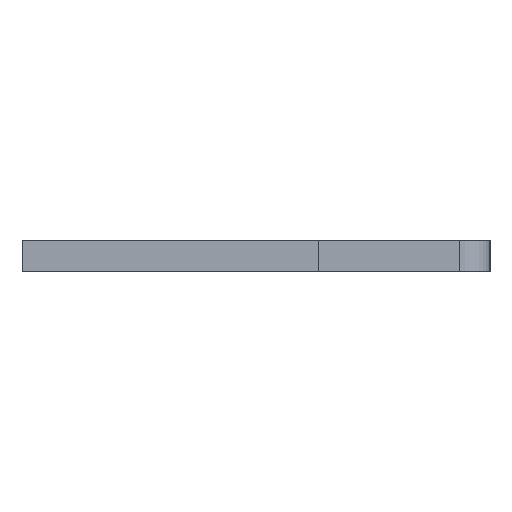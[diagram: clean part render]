
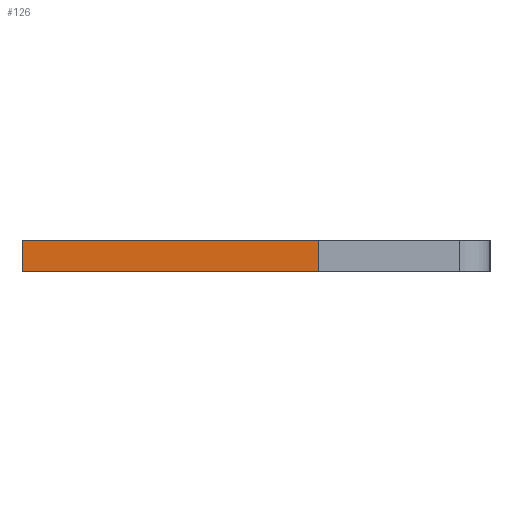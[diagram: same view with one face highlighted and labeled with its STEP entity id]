
A CAD part, left-side view. The second image highlights one B-rep face of the part: STEP entity #126.
In plain terms, the highlighted face is planar.
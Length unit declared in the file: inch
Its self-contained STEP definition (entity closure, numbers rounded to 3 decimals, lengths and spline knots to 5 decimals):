
#49 = VERTEX_POINT ( 'NONE', #751 ) ;
#65 = VECTOR ( 'NONE', #661, 39.37008 ) ;
#108 = ORIENTED_EDGE ( 'NONE', *, *, #788, .T. ) ;
#120 = PLANE ( 'NONE',  #532 ) ;
#126 = ADVANCED_FACE ( 'NONE', ( #1208 ), #120, .F. ) ;
#203 = EDGE_CURVE ( 'NONE', #691, #882, #754, .T. ) ;
#280 = CARTESIAN_POINT ( 'NONE',  ( 0.01, 0.15, -0.04 ) ) ;
#299 = CARTESIAN_POINT ( 'NONE',  ( -0.01, -0.04, -0.04 ) ) ;
#366 = ORIENTED_EDGE ( 'NONE', *, *, #372, .F. ) ;
#372 = EDGE_CURVE ( 'NONE', #1497, #882, #435, .T. ) ;
#435 = LINE ( 'NONE', #922, #771 ) ;
#532 = AXIS2_PLACEMENT_3D ( 'NONE', #910, #1214, #1453 ) ;
#661 = DIRECTION ( 'NONE',  ( 0., 1., 0. ) ) ;
#691 = VERTEX_POINT ( 'NONE', #299 ) ;
#693 = DIRECTION ( 'NONE',  ( -1., 0., 0. ) ) ;
#713 = EDGE_LOOP ( 'NONE', ( #1251, #366, #1320, #108 ) ) ;
#751 = CARTESIAN_POINT ( 'NONE',  ( 0.01, -0.04, -0.04 ) ) ;
#754 = LINE ( 'NONE', #1060, #65 ) ;
#771 = VECTOR ( 'NONE', #1466, 39.37008 ) ;
#788 = EDGE_CURVE ( 'NONE', #49, #691, #1031, .T. ) ;
#791 = LINE ( 'NONE', #280, #1117 ) ;
#812 = CARTESIAN_POINT ( 'NONE',  ( 0.01, -0.04, -0.04 ) ) ;
#826 = DIRECTION ( 'NONE',  ( 0., 1., 0. ) ) ;
#835 = EDGE_CURVE ( 'NONE', #49, #1497, #791, .T. ) ;
#882 = VERTEX_POINT ( 'NONE', #1094 ) ;
#910 = CARTESIAN_POINT ( 'NONE',  ( 0.01, 0.15, -0.04 ) ) ;
#922 = CARTESIAN_POINT ( 'NONE',  ( 0.01, 0.15, -0.04 ) ) ;
#1031 = LINE ( 'NONE', #812, #1653 ) ;
#1060 = CARTESIAN_POINT ( 'NONE',  ( -0.01, 0.15, -0.04 ) ) ;
#1094 = CARTESIAN_POINT ( 'NONE',  ( -0.01, 0.15, -0.04 ) ) ;
#1117 = VECTOR ( 'NONE', #826, 39.37008 ) ;
#1136 = CARTESIAN_POINT ( 'NONE',  ( 0.01, 0.15, -0.04 ) ) ;
#1208 = FACE_OUTER_BOUND ( 'NONE', #713, .T. ) ;
#1214 = DIRECTION ( 'NONE',  ( 0., 0., 1. ) ) ;
#1251 = ORIENTED_EDGE ( 'NONE', *, *, #203, .T. ) ;
#1320 = ORIENTED_EDGE ( 'NONE', *, *, #835, .F. ) ;
#1453 = DIRECTION ( 'NONE',  ( 1., 0., 0. ) ) ;
#1466 = DIRECTION ( 'NONE',  ( -1., 0., 0. ) ) ;
#1497 = VERTEX_POINT ( 'NONE', #1136 ) ;
#1653 = VECTOR ( 'NONE', #693, 39.37008 ) ;
